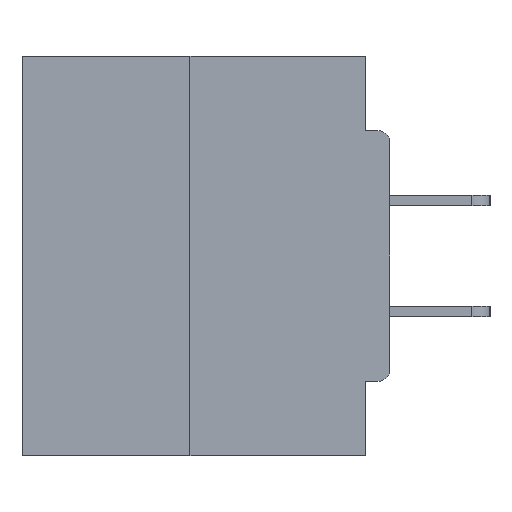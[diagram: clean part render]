
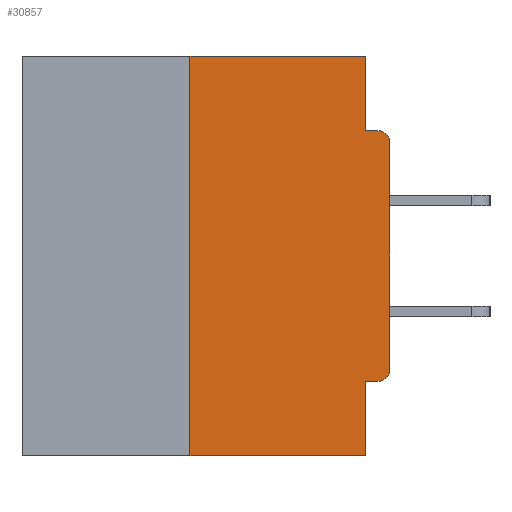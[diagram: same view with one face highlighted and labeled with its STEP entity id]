
A CAD part, left-side view. The second image highlights one B-rep face of the part: STEP entity #30857.
In plain terms, the highlighted planar face has unit normal (-1, 0, 0).
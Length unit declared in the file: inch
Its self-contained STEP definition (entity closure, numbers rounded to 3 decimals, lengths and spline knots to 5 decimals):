
#258 = VECTOR ( 'NONE', #28184, 39.37008 ) ;
#837 = CARTESIAN_POINT ( 'NONE',  ( 0., 0.031, -0.4065 ) ) ;
#1117 = CARTESIAN_POINT ( 'NONE',  ( 0., 0.031, -0.0935 ) ) ;
#1180 = CARTESIAN_POINT ( 'NONE',  ( 0., 0., 0. ) ) ;
#1943 = CIRCLE ( 'NONE', #10558, 0.015 ) ;
#2289 = CARTESIAN_POINT ( 'NONE',  ( 0., 0.015, -0.0935 ) ) ;
#2570 = ORIENTED_EDGE ( 'NONE', *, *, #14711, .T. ) ;
#2606 = VECTOR ( 'NONE', #24125, 39.37008 ) ;
#2789 = ORIENTED_EDGE ( 'NONE', *, *, #9611, .T. ) ;
#2814 = DIRECTION ( 'NONE',  ( 0., 0., 1. ) ) ;
#3004 = VECTOR ( 'NONE', #19768, 39.37008 ) ;
#3518 = ORIENTED_EDGE ( 'NONE', *, *, #16303, .F. ) ;
#4131 = EDGE_CURVE ( 'NONE', #19935, #17007, #32980, .T. ) ;
#4218 = FACE_OUTER_BOUND ( 'NONE', #8093, .T. ) ;
#4319 = ORIENTED_EDGE ( 'NONE', *, *, #4131, .F. ) ;
#5633 = CARTESIAN_POINT ( 'NONE',  ( 0., 0.25, 0. ) ) ;
#5778 = DIRECTION ( 'NONE',  ( 0., 0., -1. ) ) ;
#6823 = DIRECTION ( 'NONE',  ( -1., 0., 0. ) ) ;
#6914 = DIRECTION ( 'NONE',  ( 0., -1., 0. ) ) ;
#7127 = DIRECTION ( 'NONE',  ( 0., 0., -1. ) ) ;
#7505 = ORIENTED_EDGE ( 'NONE', *, *, #9780, .F. ) ;
#7635 = LINE ( 'NONE', #20470, #30552 ) ;
#7999 = ORIENTED_EDGE ( 'NONE', *, *, #24290, .F. ) ;
#8093 = EDGE_LOOP ( 'NONE', ( #13035, #4319, #11311, #19027, #7999, #2570, #22292, #2789, #3518, #7505 ) ) ;
#8932 = LINE ( 'NONE', #1180, #18156 ) ;
#9084 = CARTESIAN_POINT ( 'NONE',  ( 0., 0.46, 0. ) ) ;
#9326 = CARTESIAN_POINT ( 'NONE',  ( 0., 0.015, -0.1085 ) ) ;
#9611 = EDGE_CURVE ( 'NONE', #32838, #14235, #15008, .T. ) ;
#9780 = EDGE_CURVE ( 'NONE', #30124, #10861, #28861, .T. ) ;
#10558 = AXIS2_PLACEMENT_3D ( 'NONE', #30219, #27671, #7127 ) ;
#10861 = VERTEX_POINT ( 'NONE', #1117 ) ;
#11311 = ORIENTED_EDGE ( 'NONE', *, *, #17911, .T. ) ;
#11469 = DIRECTION ( 'NONE',  ( 0., 0., 1. ) ) ;
#12735 = EDGE_CURVE ( 'NONE', #14120, #24739, #33085, .T. ) ;
#13035 = ORIENTED_EDGE ( 'NONE', *, *, #22429, .F. ) ;
#14120 = VERTEX_POINT ( 'NONE', #837 ) ;
#14235 = VERTEX_POINT ( 'NONE', #2289 ) ;
#14711 = EDGE_CURVE ( 'NONE', #31932, #21094, #1943, .T. ) ;
#14984 = CARTESIAN_POINT ( 'NONE',  ( 0., 0., -0.3915 ) ) ;
#15008 = CIRCLE ( 'NONE', #17700, 0.015 ) ;
#16303 = EDGE_CURVE ( 'NONE', #10861, #14235, #25586, .T. ) ;
#16564 = CARTESIAN_POINT ( 'NONE',  ( 0., 0.031, 0. ) ) ;
#16674 = DIRECTION ( 'NONE',  ( 1., 0., 0. ) ) ;
#17007 = VERTEX_POINT ( 'NONE', #5633 ) ;
#17103 = DIRECTION ( 'NONE',  ( 0., 0., -1. ) ) ;
#17700 = AXIS2_PLACEMENT_3D ( 'NONE', #9326, #6823, #17103 ) ;
#17911 = EDGE_CURVE ( 'NONE', #19935, #24739, #22210, .T. ) ;
#18156 = VECTOR ( 'NONE', #11469, 39.37008 ) ;
#18296 = CARTESIAN_POINT ( 'NONE',  ( 0., 0.25, -0.5 ) ) ;
#18871 = CARTESIAN_POINT ( 'NONE',  ( 0., 0.46, -0.5 ) ) ;
#19027 = ORIENTED_EDGE ( 'NONE', *, *, #12735, .F. ) ;
#19423 = CARTESIAN_POINT ( 'NONE',  ( 0., 0.031, 0. ) ) ;
#19768 = DIRECTION ( 'NONE',  ( 0., -1., 0. ) ) ;
#19935 = VERTEX_POINT ( 'NONE', #18296 ) ;
#20176 = CARTESIAN_POINT ( 'NONE',  ( 0., 0.25, 0. ) ) ;
#20470 = CARTESIAN_POINT ( 'NONE',  ( 0., 0., -0.4065 ) ) ;
#20472 = CARTESIAN_POINT ( 'NONE',  ( 0., 0.031, -0.5 ) ) ;
#20976 = DIRECTION ( 'NONE',  ( 0., 1., 0. ) ) ;
#21094 = VERTEX_POINT ( 'NONE', #14984 ) ;
#22210 = LINE ( 'NONE', #18871, #2606 ) ;
#22292 = ORIENTED_EDGE ( 'NONE', *, *, #23964, .T. ) ;
#22429 = EDGE_CURVE ( 'NONE', #17007, #30124, #24653, .T. ) ;
#22468 = CARTESIAN_POINT ( 'NONE',  ( 0., 0.46, 0. ) ) ;
#23466 = CARTESIAN_POINT ( 'NONE',  ( 0., 0.031, -0.5 ) ) ;
#23964 = EDGE_CURVE ( 'NONE', #21094, #32838, #8932, .T. ) ;
#24125 = DIRECTION ( 'NONE',  ( 0., -1., 0. ) ) ;
#24290 = EDGE_CURVE ( 'NONE', #31932, #14120, #7635, .T. ) ;
#24653 = LINE ( 'NONE', #22468, #3004 ) ;
#24739 = VERTEX_POINT ( 'NONE', #23466 ) ;
#25586 = LINE ( 'NONE', #30153, #32106 ) ;
#26564 = VECTOR ( 'NONE', #2814, 39.37008 ) ;
#27266 = PLANE ( 'NONE',  #32189 ) ;
#27671 = DIRECTION ( 'NONE',  ( -1., 0., 0. ) ) ;
#28184 = DIRECTION ( 'NONE',  ( 0., 0., -1. ) ) ;
#28472 = VECTOR ( 'NONE', #5778, 39.37008 ) ;
#28861 = LINE ( 'NONE', #16564, #28472 ) ;
#29869 = CARTESIAN_POINT ( 'NONE',  ( 0., 0.015, -0.4065 ) ) ;
#30124 = VERTEX_POINT ( 'NONE', #19423 ) ;
#30153 = CARTESIAN_POINT ( 'NONE',  ( 0., 0., -0.0935 ) ) ;
#30219 = CARTESIAN_POINT ( 'NONE',  ( 0., 0.015, -0.3915 ) ) ;
#30552 = VECTOR ( 'NONE', #20976, 39.37008 ) ;
#30857 = ADVANCED_FACE ( 'NONE', ( #4218 ), #27266, .F. ) ;
#31102 = CARTESIAN_POINT ( 'NONE',  ( 0., 0., -0.1085 ) ) ;
#31932 = VERTEX_POINT ( 'NONE', #29869 ) ;
#31977 = DIRECTION ( 'NONE',  ( 0., 0., -1. ) ) ;
#32106 = VECTOR ( 'NONE', #6914, 39.37008 ) ;
#32189 = AXIS2_PLACEMENT_3D ( 'NONE', #9084, #16674, #31977 ) ;
#32838 = VERTEX_POINT ( 'NONE', #31102 ) ;
#32980 = LINE ( 'NONE', #20176, #26564 ) ;
#33085 = LINE ( 'NONE', #20472, #258 ) ;
